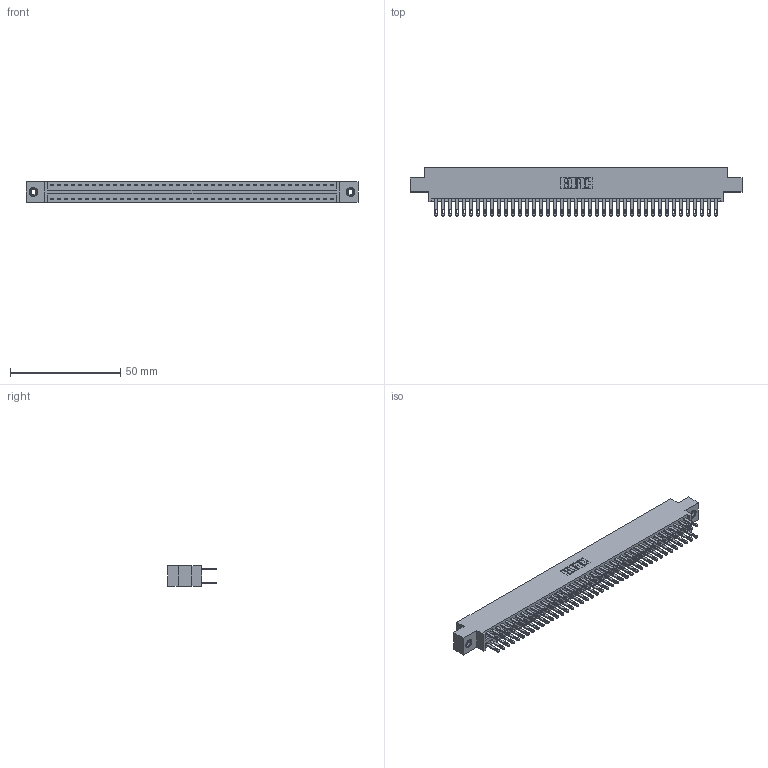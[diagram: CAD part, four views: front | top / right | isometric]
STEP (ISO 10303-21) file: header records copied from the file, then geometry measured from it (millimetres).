
FILE_DESCRIPTION (( 'STEP AP203' ), '1' );
FILE_NAME ('346-082-500-808.STEP', '2018-08-29T08:46:51', ( '' ), ( '' ), 'SwSTEP 2.0', 'SolidWorks 2016', '' );
FILE_SCHEMA (( 'CONFIG_CONTROL_DESIGN' ));
Length unit declared in the file: inch
Products named in the file (4): 346 Part_0.170 Offset - 0.156 Dia-TI; 345-292-001_345-293-100; 345-250-001_345-250-003-102; 346-082-500-808
Assembly tree (85 placements, depth 2):
  346-082-500-808
    346 Part_0.170 Offset - 0.156 Dia-TI
    345-292-001_345-293-100  x82
    345-250-001_345-250-003-102  x2
Bounding box: 150.75 x 21.84 x 9.4 mm (x, y, z)
Volume: 14781.6 mm3; surface area: 21360.5 mm2
Topology: 85 solids, 85 shells, 4122 faces, 12531 edges, 8346 vertices
Faces by surface type: plane 2490, cylinder 1616, cone 12, torus 4
Entity records: 28140 total; most frequent: CARTESIAN_POINT 4623, ORIENTED_EDGE 4550, DIRECTION 4153, EDGE_CURVE 2275, VECTOR 1955, LINE 1955, VERTEX_POINT 1512, AXIS2_PLACEMENT_3D 1099
